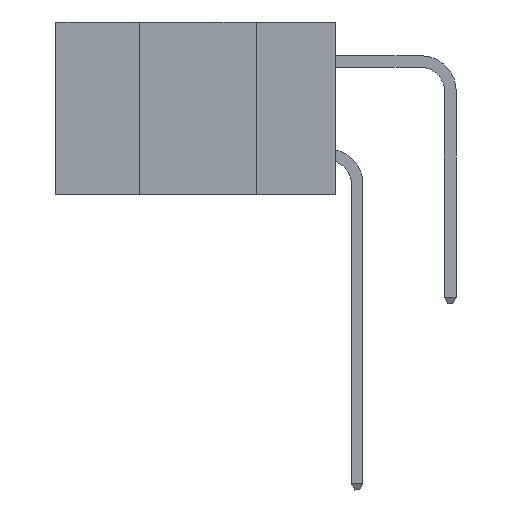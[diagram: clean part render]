
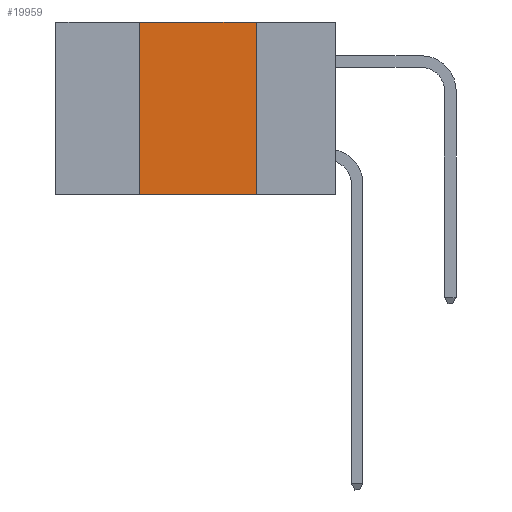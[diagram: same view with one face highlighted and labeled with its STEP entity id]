
A CAD part, left-side view. The second image highlights one B-rep face of the part: STEP entity #19959.
In plain terms, the highlighted planar face has unit normal (-1, 0, 0).
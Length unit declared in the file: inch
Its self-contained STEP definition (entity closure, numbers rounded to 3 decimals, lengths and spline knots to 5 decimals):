
#494 = LINE ( 'NONE', #14028, #10058 ) ;
#1259 = ORIENTED_EDGE ( 'NONE', *, *, #21509, .F. ) ;
#1287 = VECTOR ( 'NONE', #10743, 39.37008 ) ;
#1381 = VERTEX_POINT ( 'NONE', #17019 ) ;
#2669 = DIRECTION ( 'NONE',  ( 0., 0., -1. ) ) ;
#3880 = CARTESIAN_POINT ( 'NONE',  ( 0., 0.17, -0.37 ) ) ;
#4604 = CARTESIAN_POINT ( 'NONE',  ( 0., 0.17, 0. ) ) ;
#4698 = EDGE_CURVE ( 'NONE', #21033, #1381, #9107, .T. ) ;
#5081 = CARTESIAN_POINT ( 'NONE',  ( 0., 0.42, -0.37 ) ) ;
#6082 = VECTOR ( 'NONE', #24419, 39.37008 ) ;
#8760 = CARTESIAN_POINT ( 'NONE',  ( 0., 0.17, 0. ) ) ;
#9107 = LINE ( 'NONE', #12980, #6082 ) ;
#10058 = VECTOR ( 'NONE', #16215, 39.37008 ) ;
#10152 = LINE ( 'NONE', #17208, #1287 ) ;
#10613 = PLANE ( 'NONE',  #11214 ) ;
#10743 = DIRECTION ( 'NONE',  ( 0., -1., 0. ) ) ;
#11017 = VERTEX_POINT ( 'NONE', #3880 ) ;
#11214 = AXIS2_PLACEMENT_3D ( 'NONE', #19542, #17251, #26123 ) ;
#12980 = CARTESIAN_POINT ( 'NONE',  ( 0., 0.42, 0. ) ) ;
#13709 = VECTOR ( 'NONE', #2669, 39.37008 ) ;
#13928 = ORIENTED_EDGE ( 'NONE', *, *, #16580, .F. ) ;
#14028 = CARTESIAN_POINT ( 'NONE',  ( 0., 0.6, 0. ) ) ;
#15368 = EDGE_CURVE ( 'NONE', #21033, #11017, #10152, .T. ) ;
#16215 = DIRECTION ( 'NONE',  ( 0., -1., 0. ) ) ;
#16580 = EDGE_CURVE ( 'NONE', #1381, #17685, #494, .T. ) ;
#17019 = CARTESIAN_POINT ( 'NONE',  ( 0., 0.42, 0. ) ) ;
#17208 = CARTESIAN_POINT ( 'NONE',  ( 0., 0.6, -0.37 ) ) ;
#17251 = DIRECTION ( 'NONE',  ( 1., 0., 0. ) ) ;
#17685 = VERTEX_POINT ( 'NONE', #4604 ) ;
#18161 = LINE ( 'NONE', #8760, #13709 ) ;
#18988 = FACE_OUTER_BOUND ( 'NONE', #24215, .T. ) ;
#19542 = CARTESIAN_POINT ( 'NONE',  ( 0., 0.6, 0. ) ) ;
#19712 = ORIENTED_EDGE ( 'NONE', *, *, #15368, .T. ) ;
#19959 = ADVANCED_FACE ( 'NONE', ( #18988 ), #10613, .F. ) ;
#21033 = VERTEX_POINT ( 'NONE', #5081 ) ;
#21509 = EDGE_CURVE ( 'NONE', #17685, #11017, #18161, .T. ) ;
#24215 = EDGE_LOOP ( 'NONE', ( #1259, #13928, #27873, #19712 ) ) ;
#24419 = DIRECTION ( 'NONE',  ( 0., 0., 1. ) ) ;
#26123 = DIRECTION ( 'NONE',  ( 0., 0., -1. ) ) ;
#27873 = ORIENTED_EDGE ( 'NONE', *, *, #4698, .F. ) ;
